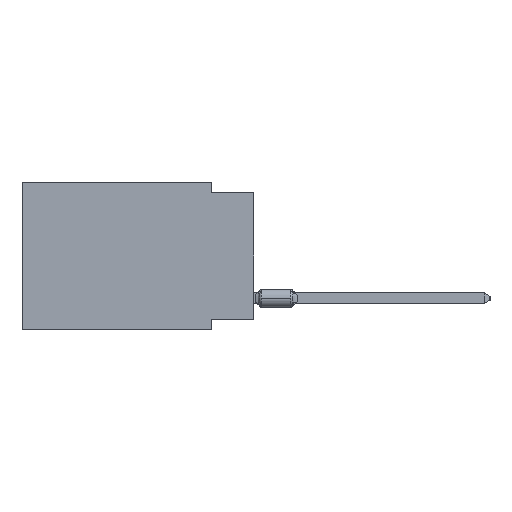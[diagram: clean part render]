
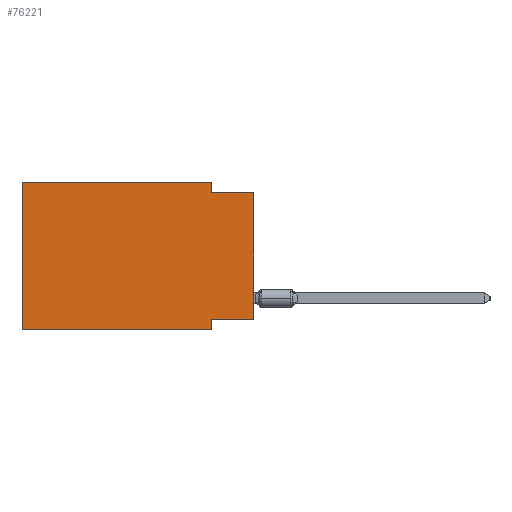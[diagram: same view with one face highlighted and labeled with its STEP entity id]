
A CAD part, left-side view. The second image highlights one B-rep face of the part: STEP entity #76221.
In plain terms, the highlighted planar face has unit normal (-1, 0, 0).
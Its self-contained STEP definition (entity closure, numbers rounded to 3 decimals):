
#117 = CARTESIAN_POINT ( 'NONE',  ( 0., 13.97, 0. ) ) ;
#419 = CARTESIAN_POINT ( 'NONE',  ( 0., 2.54, 0. ) ) ;
#2399 = EDGE_CURVE ( 'NONE', #11595, #96458, #79777, .T. ) ;
#2765 = EDGE_CURVE ( 'NONE', #27345, #96458, #54001, .T. ) ;
#3547 = DIRECTION ( 'NONE',  ( 0., -1., 0. ) ) ;
#4518 = PLANE ( 'NONE',  #79312 ) ;
#4527 = VECTOR ( 'NONE', #97761, 1000. ) ;
#4758 = VECTOR ( 'NONE', #44130, 1000. ) ;
#9940 = EDGE_CURVE ( 'NONE', #83378, #110967, #46528, .T. ) ;
#10477 = VECTOR ( 'NONE', #61031, 1000. ) ;
#11595 = VERTEX_POINT ( 'NONE', #40141 ) ;
#12734 = ORIENTED_EDGE ( 'NONE', *, *, #61083, .F. ) ;
#13232 = ORIENTED_EDGE ( 'NONE', *, *, #72519, .F. ) ;
#17845 = VECTOR ( 'NONE', #105996, 1000. ) ;
#17940 = CARTESIAN_POINT ( 'NONE',  ( 0., 2.54, -0.635 ) ) ;
#19016 = ORIENTED_EDGE ( 'NONE', *, *, #58272, .F. ) ;
#19146 = ORIENTED_EDGE ( 'NONE', *, *, #2765, .F. ) ;
#26516 = DIRECTION ( 'NONE',  ( 0., 0., -1. ) ) ;
#26918 = LINE ( 'NONE', #69313, #4758 ) ;
#27345 = VERTEX_POINT ( 'NONE', #59821 ) ;
#30335 = ORIENTED_EDGE ( 'NONE', *, *, #49736, .F. ) ;
#35738 = CARTESIAN_POINT ( 'NONE',  ( 0., 2.54, -8.89 ) ) ;
#40141 = CARTESIAN_POINT ( 'NONE',  ( 0., 13.97, -8.89 ) ) ;
#40581 = DIRECTION ( 'NONE',  ( 1., 0., 0. ) ) ;
#41142 = DIRECTION ( 'NONE',  ( 0., 0., -1. ) ) ;
#43591 = LINE ( 'NONE', #78521, #17845 ) ;
#44130 = DIRECTION ( 'NONE',  ( 0., 0., 1. ) ) ;
#44884 = LINE ( 'NONE', #98105, #76206 ) ;
#46023 = DIRECTION ( 'NONE',  ( 0., -1., 0. ) ) ;
#46528 = LINE ( 'NONE', #91131, #10477 ) ;
#46553 = DIRECTION ( 'NONE',  ( 0., -1., 0. ) ) ;
#47998 = VERTEX_POINT ( 'NONE', #17940 ) ;
#49077 = ORIENTED_EDGE ( 'NONE', *, *, #2399, .T. ) ;
#49735 = FACE_OUTER_BOUND ( 'NONE', #81299, .T. ) ;
#49736 = EDGE_CURVE ( 'NONE', #52529, #47998, #43591, .T. ) ;
#52529 = VERTEX_POINT ( 'NONE', #419 ) ;
#53116 = CARTESIAN_POINT ( 'NONE',  ( 0., 0., -8.255 ) ) ;
#54001 = LINE ( 'NONE', #88352, #98124 ) ;
#54094 = ORIENTED_EDGE ( 'NONE', *, *, #84532, .F. ) ;
#55014 = CARTESIAN_POINT ( 'NONE',  ( 0., 0., -8.255 ) ) ;
#56676 = CARTESIAN_POINT ( 'NONE',  ( 0., 0., -0.635 ) ) ;
#56736 = VECTOR ( 'NONE', #3547, 1000. ) ;
#58272 = EDGE_CURVE ( 'NONE', #83378, #27345, #105209, .T. ) ;
#59821 = CARTESIAN_POINT ( 'NONE',  ( 0., 2.54, -8.255 ) ) ;
#61031 = DIRECTION ( 'NONE',  ( 0., 0., 1. ) ) ;
#61083 = EDGE_CURVE ( 'NONE', #11595, #66942, #26918, .T. ) ;
#64810 = CARTESIAN_POINT ( 'NONE',  ( 0., 13.97, 0. ) ) ;
#66942 = VERTEX_POINT ( 'NONE', #117 ) ;
#67411 = ORIENTED_EDGE ( 'NONE', *, *, #9940, .T. ) ;
#69313 = CARTESIAN_POINT ( 'NONE',  ( 0., 13.97, 0. ) ) ;
#72519 = EDGE_CURVE ( 'NONE', #66942, #52529, #101407, .T. ) ;
#76206 = VECTOR ( 'NONE', #46023, 1000. ) ;
#76221 = ADVANCED_FACE ( 'NONE', ( #49735 ), #4518, .F. ) ;
#78521 = CARTESIAN_POINT ( 'NONE',  ( 0., 2.54, 0. ) ) ;
#79312 = AXIS2_PLACEMENT_3D ( 'NONE', #101800, #40581, #41142 ) ;
#79777 = LINE ( 'NONE', #89502, #101673 ) ;
#81299 = EDGE_LOOP ( 'NONE', ( #67411, #54094, #30335, #13232, #12734, #49077, #19146, #19016 ) ) ;
#83378 = VERTEX_POINT ( 'NONE', #55014 ) ;
#84532 = EDGE_CURVE ( 'NONE', #47998, #110967, #44884, .T. ) ;
#88352 = CARTESIAN_POINT ( 'NONE',  ( 0., 2.54, -8.89 ) ) ;
#89502 = CARTESIAN_POINT ( 'NONE',  ( 0., 13.97, -8.89 ) ) ;
#91131 = CARTESIAN_POINT ( 'NONE',  ( 0., 0., 0. ) ) ;
#96458 = VERTEX_POINT ( 'NONE', #35738 ) ;
#97761 = DIRECTION ( 'NONE',  ( 0., 1., 0. ) ) ;
#98105 = CARTESIAN_POINT ( 'NONE',  ( 0., 0., -0.635 ) ) ;
#98124 = VECTOR ( 'NONE', #26516, 1000. ) ;
#101407 = LINE ( 'NONE', #64810, #56736 ) ;
#101673 = VECTOR ( 'NONE', #46553, 1000. ) ;
#101800 = CARTESIAN_POINT ( 'NONE',  ( 0., 13.97, 0. ) ) ;
#105209 = LINE ( 'NONE', #53116, #4527 ) ;
#105996 = DIRECTION ( 'NONE',  ( 0., 0., -1. ) ) ;
#110967 = VERTEX_POINT ( 'NONE', #56676 ) ;
